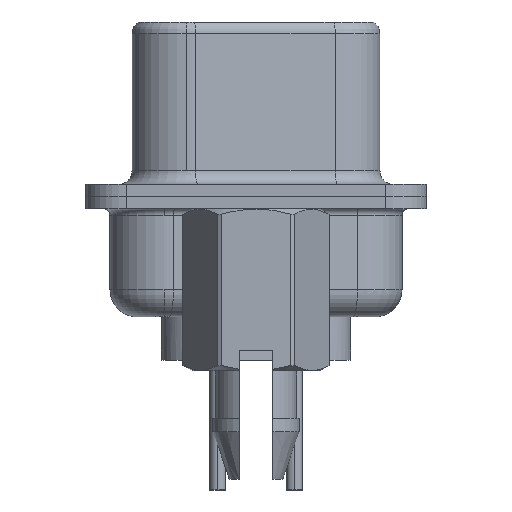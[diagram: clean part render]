
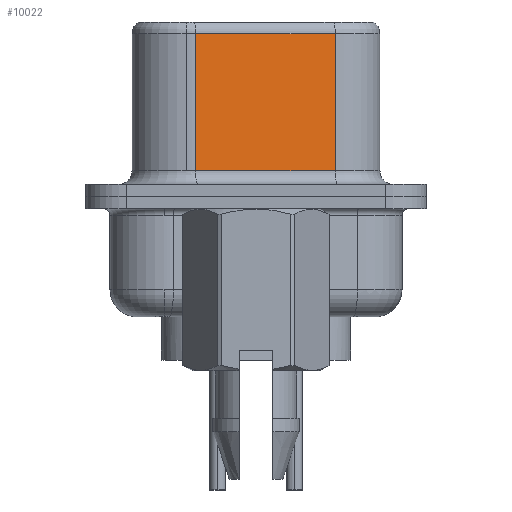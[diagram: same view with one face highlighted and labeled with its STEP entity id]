
A CAD part, left-side view. The second image highlights one B-rep face of the part: STEP entity #10022.
In plain terms, the highlighted planar face has unit normal (-0.985, -0.174, 0).
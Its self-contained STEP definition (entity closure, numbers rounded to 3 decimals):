
#621 = FACE_OUTER_BOUND ( 'NONE', #5809, .T. ) ;
#1302 = LINE ( 'NONE', #22369, #5325 ) ;
#1303 = VERTEX_POINT ( 'NONE', #20159 ) ;
#2027 = VECTOR ( 'NONE', #16793, 1000. ) ;
#2447 = CARTESIAN_POINT ( 'NONE',  ( 4.575, -2.927, 6.52 ) ) ;
#2477 = DIRECTION ( 'NONE',  ( 0., 0., -1. ) ) ;
#2565 = EDGE_CURVE ( 'NONE', #13778, #22388, #13522, .T. ) ;
#2589 = CARTESIAN_POINT ( 'NONE',  ( 3.665, 2.233, 6.52 ) ) ;
#2898 = VECTOR ( 'NONE', #15189, 1000. ) ;
#3848 = LINE ( 'NONE', #2589, #10024 ) ;
#4905 = ORIENTED_EDGE ( 'NONE', *, *, #14708, .T. ) ;
#5325 = VECTOR ( 'NONE', #21195, 1000. ) ;
#5809 = EDGE_LOOP ( 'NONE', ( #21936, #22359, #18443, #4905 ) ) ;
#6265 = CARTESIAN_POINT ( 'NONE',  ( 4.575, -2.927, 6.02 ) ) ;
#6853 = EDGE_CURVE ( 'NONE', #13778, #9850, #22106, .T. ) ;
#7037 = AXIS2_PLACEMENT_3D ( 'NONE', #2447, #7595, #14653 ) ;
#7595 = DIRECTION ( 'NONE',  ( 0.985, 0.174, 0. ) ) ;
#8392 = CARTESIAN_POINT ( 'NONE',  ( 3.665, 2.233, 6.02 ) ) ;
#9850 = VERTEX_POINT ( 'NONE', #19409 ) ;
#10022 = ADVANCED_FACE ( 'NONE', ( #621 ), #18043, .F. ) ;
#10024 = VECTOR ( 'NONE', #2477, 1000. ) ;
#13522 = LINE ( 'NONE', #18594, #2027 ) ;
#13778 = VERTEX_POINT ( 'NONE', #6265 ) ;
#14653 = DIRECTION ( 'NONE',  ( -0.174, 0.985, 0. ) ) ;
#14708 = EDGE_CURVE ( 'NONE', #1303, #9850, #1302, .T. ) ;
#15189 = DIRECTION ( 'NONE',  ( 0., 0., -1. ) ) ;
#16793 = DIRECTION ( 'NONE',  ( -0.174, 0.985, 0. ) ) ;
#18043 = PLANE ( 'NONE',  #7037 ) ;
#18443 = ORIENTED_EDGE ( 'NONE', *, *, #19007, .T. ) ;
#18594 = CARTESIAN_POINT ( 'NONE',  ( 4.575, -2.927, 6.02 ) ) ;
#19007 = EDGE_CURVE ( 'NONE', #22388, #1303, #3848, .T. ) ;
#19409 = CARTESIAN_POINT ( 'NONE',  ( 4.575, -2.927, 0.95 ) ) ;
#20159 = CARTESIAN_POINT ( 'NONE',  ( 3.665, 2.233, 0.95 ) ) ;
#20505 = CARTESIAN_POINT ( 'NONE',  ( 4.575, -2.927, 6.52 ) ) ;
#21195 = DIRECTION ( 'NONE',  ( 0.174, -0.985, 0. ) ) ;
#21936 = ORIENTED_EDGE ( 'NONE', *, *, #6853, .F. ) ;
#22106 = LINE ( 'NONE', #20505, #2898 ) ;
#22359 = ORIENTED_EDGE ( 'NONE', *, *, #2565, .T. ) ;
#22369 = CARTESIAN_POINT ( 'NONE',  ( 4.575, -2.927, 0.95 ) ) ;
#22388 = VERTEX_POINT ( 'NONE', #8392 ) ;
